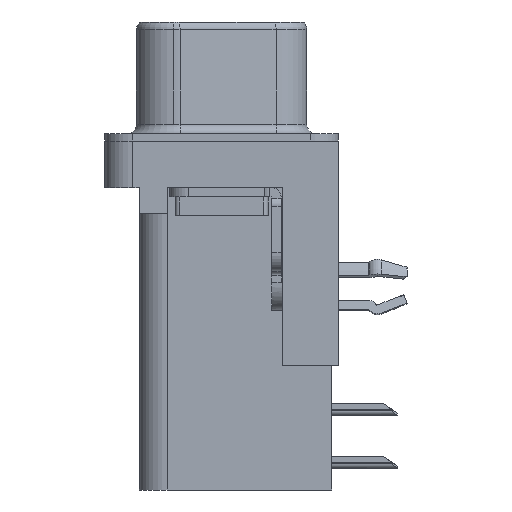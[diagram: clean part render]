
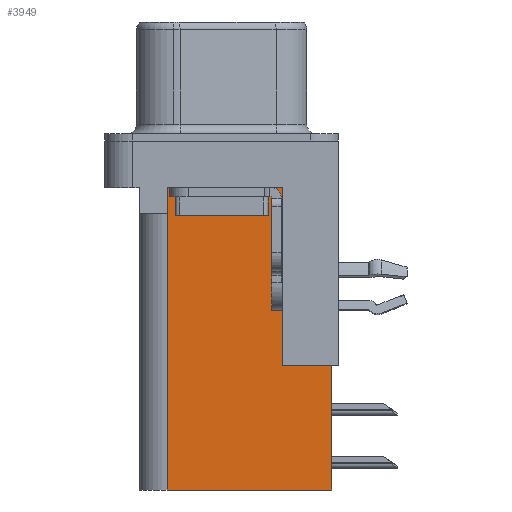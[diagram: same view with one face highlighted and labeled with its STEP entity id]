
A CAD part, left-side view. The second image highlights one B-rep face of the part: STEP entity #3949.
In plain terms, the highlighted planar face has unit normal (-1, 0, 0).
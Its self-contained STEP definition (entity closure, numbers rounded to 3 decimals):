
#76 = EDGE_CURVE ( 'NONE', #405, #7155, #12908, .T. ) ;
#122 = CARTESIAN_POINT ( 'NONE',  ( 3.7, -3.295, -2.5 ) ) ;
#315 = EDGE_CURVE ( 'NONE', #7155, #8263, #11913, .T. ) ;
#405 = VERTEX_POINT ( 'NONE', #8104 ) ;
#595 = VECTOR ( 'NONE', #9495, 1000. ) ;
#717 = DIRECTION ( 'NONE',  ( 0., 1., 0. ) ) ;
#799 = LINE ( 'NONE', #12912, #595 ) ;
#1765 = CARTESIAN_POINT ( 'NONE',  ( 3.7, 2.925, -18.76 ) ) ;
#3141 = ORIENTED_EDGE ( 'NONE', *, *, #4210, .F. ) ;
#3612 = EDGE_CURVE ( 'NONE', #14328, #10006, #18324, .T. ) ;
#3662 = CARTESIAN_POINT ( 'NONE',  ( 3.7, 2.895, -2.5 ) ) ;
#3949 = ADVANCED_FACE ( 'NONE', ( #16669 ), #22152, .F. ) ;
#4194 = ORIENTED_EDGE ( 'NONE', *, *, #76, .T. ) ;
#4210 = EDGE_CURVE ( 'NONE', #405, #6747, #15416, .T. ) ;
#5923 = VECTOR ( 'NONE', #17700, 1000. ) ;
#5990 = LINE ( 'NONE', #15999, #5923 ) ;
#6455 = LINE ( 'NONE', #11012, #7443 ) ;
#6747 = VERTEX_POINT ( 'NONE', #19907 ) ;
#7155 = VERTEX_POINT ( 'NONE', #11219 ) ;
#7417 = DIRECTION ( 'NONE',  ( 0., 1., 0. ) ) ;
#7443 = VECTOR ( 'NONE', #19442, 1000. ) ;
#7536 = EDGE_CURVE ( 'NONE', #10006, #21962, #799, .T. ) ;
#7671 = DIRECTION ( 'NONE',  ( 1., 0., 0. ) ) ;
#8104 = CARTESIAN_POINT ( 'NONE',  ( 3.7, -5.925, -12.05 ) ) ;
#8263 = VERTEX_POINT ( 'NONE', #9257 ) ;
#8619 = CARTESIAN_POINT ( 'NONE',  ( 3.7, 2.895, -3.9 ) ) ;
#8700 = CARTESIAN_POINT ( 'NONE',  ( 3.7, 2.895, -3.9 ) ) ;
#9144 = DIRECTION ( 'NONE',  ( 0., 0., -1. ) ) ;
#9224 = DIRECTION ( 'NONE',  ( 0., 0., 1. ) ) ;
#9257 = CARTESIAN_POINT ( 'NONE',  ( 3.7, -3.295, -2.5 ) ) ;
#9495 = DIRECTION ( 'NONE',  ( 0., 1., 0. ) ) ;
#10006 = VERTEX_POINT ( 'NONE', #8619 ) ;
#10650 = CARTESIAN_POINT ( 'NONE',  ( 3.7, -3.295, -18.76 ) ) ;
#11012 = CARTESIAN_POINT ( 'NONE',  ( 3.7, 2.925, -18.76 ) ) ;
#11219 = CARTESIAN_POINT ( 'NONE',  ( 3.7, -3.295, -12.05 ) ) ;
#11256 = VECTOR ( 'NONE', #20783, 1000. ) ;
#11328 = LINE ( 'NONE', #122, #11256 ) ;
#11741 = ORIENTED_EDGE ( 'NONE', *, *, #15438, .F. ) ;
#11889 = VECTOR ( 'NONE', #9224, 1000. ) ;
#11913 = LINE ( 'NONE', #10650, #11889 ) ;
#12678 = VECTOR ( 'NONE', #717, 1000. ) ;
#12770 = DIRECTION ( 'NONE',  ( 0., 0., -1. ) ) ;
#12908 = LINE ( 'NONE', #19627, #12678 ) ;
#12912 = CARTESIAN_POINT ( 'NONE',  ( 3.7, 0., -3.9 ) ) ;
#13627 = ORIENTED_EDGE ( 'NONE', *, *, #3612, .T. ) ;
#13856 = CARTESIAN_POINT ( 'NONE',  ( 3.7, -3.295, -18.76 ) ) ;
#14328 = VERTEX_POINT ( 'NONE', #3662 ) ;
#14709 = CARTESIAN_POINT ( 'NONE',  ( 3.7, 2.925, -3.9 ) ) ;
#15372 = VECTOR ( 'NONE', #9144, 1000. ) ;
#15416 = LINE ( 'NONE', #15717, #15372 ) ;
#15438 = EDGE_CURVE ( 'NONE', #21645, #21962, #6455, .T. ) ;
#15463 = EDGE_LOOP ( 'NONE', ( #18707, #13627, #17279, #11741, #15652, #3141, #4194, #17957 ) ) ;
#15652 = ORIENTED_EDGE ( 'NONE', *, *, #21836, .F. ) ;
#15717 = CARTESIAN_POINT ( 'NONE',  ( 3.7, -5.925, -2. ) ) ;
#15999 = CARTESIAN_POINT ( 'NONE',  ( 3.7, -3.295, -18.76 ) ) ;
#16669 = FACE_OUTER_BOUND ( 'NONE', #15463, .T. ) ;
#17279 = ORIENTED_EDGE ( 'NONE', *, *, #7536, .T. ) ;
#17700 = DIRECTION ( 'NONE',  ( 0., 1., 0. ) ) ;
#17957 = ORIENTED_EDGE ( 'NONE', *, *, #315, .T. ) ;
#18144 = VECTOR ( 'NONE', #12770, 1000. ) ;
#18324 = LINE ( 'NONE', #8700, #18144 ) ;
#18400 = AXIS2_PLACEMENT_3D ( 'NONE', #13856, #7671, #7417 ) ;
#18707 = ORIENTED_EDGE ( 'NONE', *, *, #20085, .T. ) ;
#19442 = DIRECTION ( 'NONE',  ( 0., 0., 1. ) ) ;
#19627 = CARTESIAN_POINT ( 'NONE',  ( 3.7, -6.295, -12.05 ) ) ;
#19907 = CARTESIAN_POINT ( 'NONE',  ( 3.7, -5.925, -18.76 ) ) ;
#20085 = EDGE_CURVE ( 'NONE', #8263, #14328, #11328, .T. ) ;
#20783 = DIRECTION ( 'NONE',  ( 0., 1., 0. ) ) ;
#21645 = VERTEX_POINT ( 'NONE', #1765 ) ;
#21836 = EDGE_CURVE ( 'NONE', #6747, #21645, #5990, .T. ) ;
#21962 = VERTEX_POINT ( 'NONE', #14709 ) ;
#22152 = PLANE ( 'NONE',  #18400 ) ;
